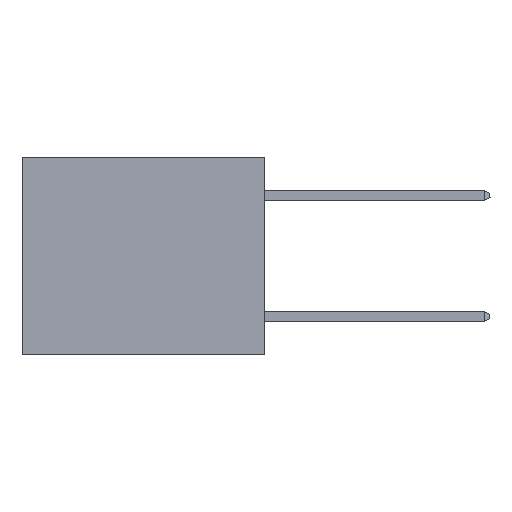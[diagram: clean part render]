
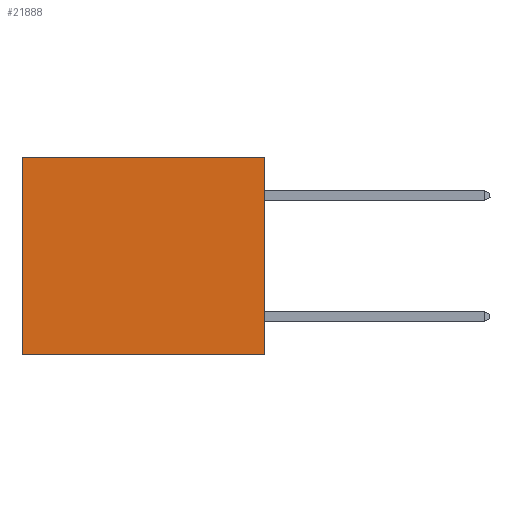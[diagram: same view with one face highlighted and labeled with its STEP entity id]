
A CAD part, left-side view. The second image highlights one B-rep face of the part: STEP entity #21888.
In plain terms, the highlighted planar face has unit normal (-1, 0, 0).
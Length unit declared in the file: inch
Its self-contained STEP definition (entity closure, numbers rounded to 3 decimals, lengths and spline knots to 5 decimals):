
#1796 = VECTOR ( 'NONE', #17799, 39.37008 ) ;
#3338 = CARTESIAN_POINT ( 'NONE',  ( 0.3165, 0., -0.49 ) ) ;
#3394 = CARTESIAN_POINT ( 'NONE',  ( 0.3165, 0., -0.49 ) ) ;
#3736 = EDGE_CURVE ( 'NONE', #11346, #17675, #12865, .T. ) ;
#4156 = EDGE_CURVE ( 'NONE', #8722, #20276, #8511, .T. ) ;
#5763 = EDGE_CURVE ( 'NONE', #8722, #11346, #19736, .T. ) ;
#5908 = AXIS2_PLACEMENT_3D ( 'NONE', #3394, #7155, #12830 ) ;
#6451 = ORIENTED_EDGE ( 'NONE', *, *, #11392, .F. ) ;
#7155 = DIRECTION ( 'NONE',  ( 1., 0., 0. ) ) ;
#7380 = CARTESIAN_POINT ( 'NONE',  ( 0.3165, 0., -0.49 ) ) ;
#7717 = EDGE_LOOP ( 'NONE', ( #14696, #6451, #17175, #8158 ) ) ;
#8158 = ORIENTED_EDGE ( 'NONE', *, *, #5763, .T. ) ;
#8511 = LINE ( 'NONE', #7380, #15744 ) ;
#8538 = DIRECTION ( 'NONE',  ( 0., 1., 0. ) ) ;
#8722 = VERTEX_POINT ( 'NONE', #18218 ) ;
#10313 = CARTESIAN_POINT ( 'NONE',  ( 0.3165, 0.6, -0.49 ) ) ;
#10677 = CARTESIAN_POINT ( 'NONE',  ( 0.3165, 0., -0.49 ) ) ;
#10830 = CARTESIAN_POINT ( 'NONE',  ( 0.3165, 0.6, 0. ) ) ;
#11346 = VERTEX_POINT ( 'NONE', #10830 ) ;
#11392 = EDGE_CURVE ( 'NONE', #20276, #17675, #13224, .T. ) ;
#12786 = CARTESIAN_POINT ( 'NONE',  ( 0.3165, 0., 0. ) ) ;
#12830 = DIRECTION ( 'NONE',  ( 0., 0., -1. ) ) ;
#12865 = LINE ( 'NONE', #15887, #21462 ) ;
#13224 = LINE ( 'NONE', #3338, #20215 ) ;
#14696 = ORIENTED_EDGE ( 'NONE', *, *, #3736, .T. ) ;
#15744 = VECTOR ( 'NONE', #21231, 39.37008 ) ;
#15887 = CARTESIAN_POINT ( 'NONE',  ( 0.3165, 0.6, -0.49 ) ) ;
#17175 = ORIENTED_EDGE ( 'NONE', *, *, #4156, .F. ) ;
#17675 = VERTEX_POINT ( 'NONE', #10313 ) ;
#17799 = DIRECTION ( 'NONE',  ( 0., 1., 0. ) ) ;
#18218 = CARTESIAN_POINT ( 'NONE',  ( 0.3165, 0., 0. ) ) ;
#18745 = PLANE ( 'NONE',  #5908 ) ;
#19260 = DIRECTION ( 'NONE',  ( 0., 0., -1. ) ) ;
#19736 = LINE ( 'NONE', #12786, #1796 ) ;
#20215 = VECTOR ( 'NONE', #8538, 39.37008 ) ;
#20276 = VERTEX_POINT ( 'NONE', #10677 ) ;
#21231 = DIRECTION ( 'NONE',  ( 0., 0., -1. ) ) ;
#21462 = VECTOR ( 'NONE', #19260, 39.37008 ) ;
#21734 = FACE_OUTER_BOUND ( 'NONE', #7717, .T. ) ;
#21888 = ADVANCED_FACE ( 'NONE', ( #21734 ), #18745, .F. ) ;
